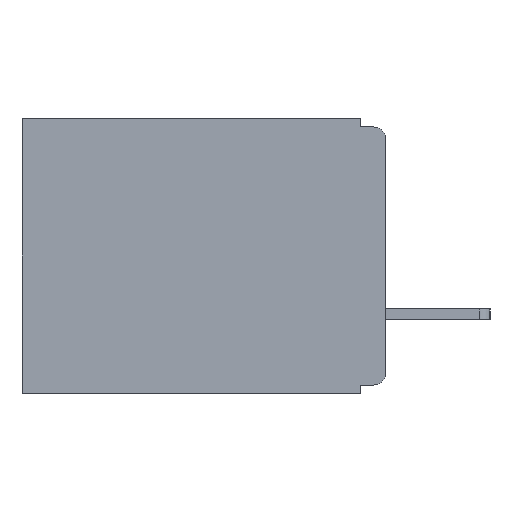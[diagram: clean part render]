
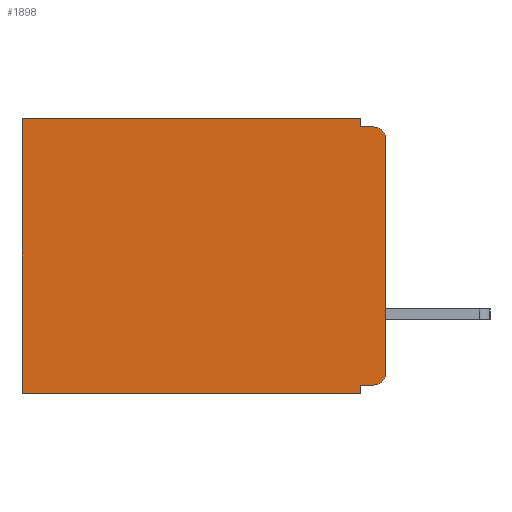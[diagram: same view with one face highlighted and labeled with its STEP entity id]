
A CAD part, left-side view. The second image highlights one B-rep face of the part: STEP entity #1898.
In plain terms, the highlighted planar face has unit normal (-1, 0, 0).
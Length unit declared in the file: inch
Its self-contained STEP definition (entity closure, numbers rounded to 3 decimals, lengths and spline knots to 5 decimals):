
#251 = DIRECTION ( 'NONE',  ( 0., 0., -1. ) ) ;
#372 = ORIENTED_EDGE ( 'NONE', *, *, #12766, .F. ) ;
#393 = ORIENTED_EDGE ( 'NONE', *, *, #17634, .T. ) ;
#394 = DIRECTION ( 'NONE',  ( -1., 0., 0. ) ) ;
#503 = CARTESIAN_POINT ( 'NONE',  ( 0.3, 0.015, -0.01 ) ) ;
#711 = EDGE_CURVE ( 'NONE', #5942, #2890, #13595, .T. ) ;
#761 = EDGE_LOOP ( 'NONE', ( #372, #393, #16318, #6974, #11481, #6642, #2653, #2549, #3248, #4195 ) ) ;
#895 = CARTESIAN_POINT ( 'NONE',  ( 0.3, 0.015, -0.025 ) ) ;
#1538 = VECTOR ( 'NONE', #16072, 39.37008 ) ;
#1556 = LINE ( 'NONE', #17189, #1538 ) ;
#1898 = ADVANCED_FACE ( 'NONE', ( #4660 ), #11529, .F. ) ;
#2549 = ORIENTED_EDGE ( 'NONE', *, *, #15947, .F. ) ;
#2653 = ORIENTED_EDGE ( 'NONE', *, *, #11017, .F. ) ;
#2890 = VERTEX_POINT ( 'NONE', #8031 ) ;
#3248 = ORIENTED_EDGE ( 'NONE', *, *, #13412, .F. ) ;
#3518 = VERTEX_POINT ( 'NONE', #6288 ) ;
#3799 = VERTEX_POINT ( 'NONE', #11027 ) ;
#3933 = CARTESIAN_POINT ( 'NONE',  ( 0.3, 0.031, 0. ) ) ;
#4195 = ORIENTED_EDGE ( 'NONE', *, *, #11615, .T. ) ;
#4516 = VECTOR ( 'NONE', #8442, 39.37008 ) ;
#4660 = FACE_OUTER_BOUND ( 'NONE', #761, .T. ) ;
#4702 = VERTEX_POINT ( 'NONE', #17756 ) ;
#4814 = VERTEX_POINT ( 'NONE', #14777 ) ;
#5022 = CARTESIAN_POINT ( 'NONE',  ( 0.3, 0., -0.305 ) ) ;
#5296 = LINE ( 'NONE', #8499, #4516 ) ;
#5942 = VERTEX_POINT ( 'NONE', #17124 ) ;
#5994 = VECTOR ( 'NONE', #14035, 39.37008 ) ;
#6066 = LINE ( 'NONE', #15527, #5994 ) ;
#6288 = CARTESIAN_POINT ( 'NONE',  ( 0.3, 0.031, -0.33 ) ) ;
#6588 = AXIS2_PLACEMENT_3D ( 'NONE', #895, #394, #251 ) ;
#6642 = ORIENTED_EDGE ( 'NONE', *, *, #711, .T. ) ;
#6738 = VERTEX_POINT ( 'NONE', #3933 ) ;
#6875 = DIRECTION ( 'NONE',  ( 1., 0., 0. ) ) ;
#6974 = ORIENTED_EDGE ( 'NONE', *, *, #14761, .F. ) ;
#7471 = CARTESIAN_POINT ( 'NONE',  ( 0.3, 0., -0.33 ) ) ;
#8031 = CARTESIAN_POINT ( 'NONE',  ( 0.3, 0.437, -0.33 ) ) ;
#8080 = DIRECTION ( 'NONE',  ( 0., 0., -1. ) ) ;
#8122 = DIRECTION ( 'NONE',  ( 0., 1., 0. ) ) ;
#8213 = CARTESIAN_POINT ( 'NONE',  ( 0.3, 0.031, 0. ) ) ;
#8396 = EDGE_CURVE ( 'NONE', #4702, #13288, #5296, .T. ) ;
#8442 = DIRECTION ( 'NONE',  ( 0., -1., 0. ) ) ;
#8499 = CARTESIAN_POINT ( 'NONE',  ( 0.3, 0., -0.01 ) ) ;
#8586 = VECTOR ( 'NONE', #13148, 39.37008 ) ;
#8629 = LINE ( 'NONE', #13050, #8586 ) ;
#9984 = VERTEX_POINT ( 'NONE', #10643 ) ;
#10643 = CARTESIAN_POINT ( 'NONE',  ( 0.3, 0., -0.025 ) ) ;
#10718 = AXIS2_PLACEMENT_3D ( 'NONE', #14571, #6875, #17483 ) ;
#11017 = EDGE_CURVE ( 'NONE', #3518, #2890, #17859, .T. ) ;
#11027 = CARTESIAN_POINT ( 'NONE',  ( 0.3, 0.031, -0.32 ) ) ;
#11481 = ORIENTED_EDGE ( 'NONE', *, *, #11587, .T. ) ;
#11515 = AXIS2_PLACEMENT_3D ( 'NONE', #16361, #16317, #16223 ) ;
#11529 = PLANE ( 'NONE',  #10718 ) ;
#11587 = EDGE_CURVE ( 'NONE', #6738, #5942, #13150, .T. ) ;
#11615 = EDGE_CURVE ( 'NONE', #4814, #16105, #13035, .T. ) ;
#11924 = CIRCLE ( 'NONE', #6588, 0.015 ) ;
#12766 = EDGE_CURVE ( 'NONE', #9984, #16105, #8629, .T. ) ;
#12790 = VECTOR ( 'NONE', #8080, 39.37008 ) ;
#13035 = CIRCLE ( 'NONE', #11515, 0.015 ) ;
#13050 = CARTESIAN_POINT ( 'NONE',  ( 0.3, 0., -0.33 ) ) ;
#13072 = LINE ( 'NONE', #8213, #12790 ) ;
#13076 = VECTOR ( 'NONE', #16973, 39.37008 ) ;
#13148 = DIRECTION ( 'NONE',  ( 0., 0., -1. ) ) ;
#13150 = LINE ( 'NONE', #17020, #13076 ) ;
#13288 = VERTEX_POINT ( 'NONE', #503 ) ;
#13412 = EDGE_CURVE ( 'NONE', #4814, #3799, #6066, .T. ) ;
#13559 = VECTOR ( 'NONE', #17663, 39.37008 ) ;
#13595 = LINE ( 'NONE', #17176, #13559 ) ;
#14035 = DIRECTION ( 'NONE',  ( 0., 1., 0. ) ) ;
#14571 = CARTESIAN_POINT ( 'NONE',  ( 0.3, 0., -0.33 ) ) ;
#14761 = EDGE_CURVE ( 'NONE', #6738, #4702, #13072, .T. ) ;
#14777 = CARTESIAN_POINT ( 'NONE',  ( 0.3, 0.015, -0.32 ) ) ;
#15527 = CARTESIAN_POINT ( 'NONE',  ( 0.3, 0., -0.32 ) ) ;
#15947 = EDGE_CURVE ( 'NONE', #3799, #3518, #1556, .T. ) ;
#16072 = DIRECTION ( 'NONE',  ( 0., 0., -1. ) ) ;
#16105 = VERTEX_POINT ( 'NONE', #5022 ) ;
#16223 = DIRECTION ( 'NONE',  ( 0., 0., -1. ) ) ;
#16317 = DIRECTION ( 'NONE',  ( -1., 0., 0. ) ) ;
#16318 = ORIENTED_EDGE ( 'NONE', *, *, #8396, .F. ) ;
#16361 = CARTESIAN_POINT ( 'NONE',  ( 0.3, 0.015, -0.305 ) ) ;
#16973 = DIRECTION ( 'NONE',  ( 0., 1., 0. ) ) ;
#17020 = CARTESIAN_POINT ( 'NONE',  ( 0.3, 0., 0. ) ) ;
#17124 = CARTESIAN_POINT ( 'NONE',  ( 0.3, 0.437, 0. ) ) ;
#17169 = VECTOR ( 'NONE', #8122, 39.37008 ) ;
#17176 = CARTESIAN_POINT ( 'NONE',  ( 0.3, 0.437, -0.33 ) ) ;
#17189 = CARTESIAN_POINT ( 'NONE',  ( 0.3, 0.031, -0.33 ) ) ;
#17483 = DIRECTION ( 'NONE',  ( 0., 0., -1. ) ) ;
#17634 = EDGE_CURVE ( 'NONE', #9984, #13288, #11924, .T. ) ;
#17663 = DIRECTION ( 'NONE',  ( 0., 0., -1. ) ) ;
#17756 = CARTESIAN_POINT ( 'NONE',  ( 0.3, 0.031, -0.01 ) ) ;
#17859 = LINE ( 'NONE', #7471, #17169 ) ;
